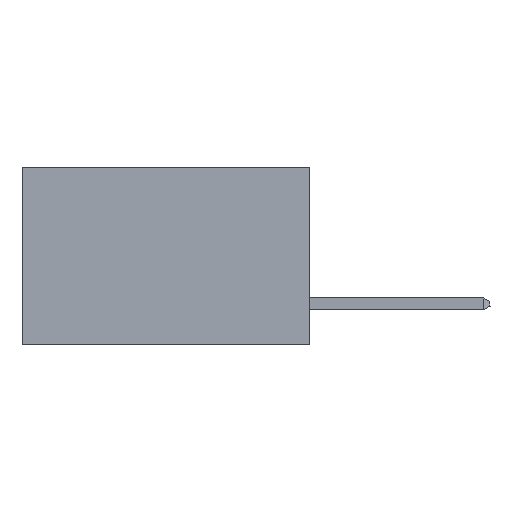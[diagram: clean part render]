
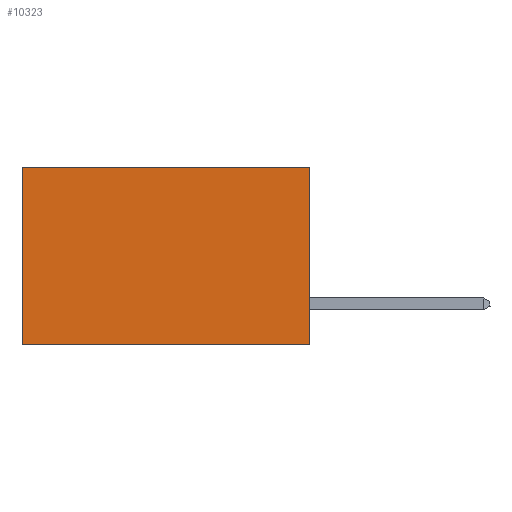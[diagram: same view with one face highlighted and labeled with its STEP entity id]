
A CAD part, left-side view. The second image highlights one B-rep face of the part: STEP entity #10323.
In plain terms, the highlighted planar face has unit normal (-1, 0, 0).
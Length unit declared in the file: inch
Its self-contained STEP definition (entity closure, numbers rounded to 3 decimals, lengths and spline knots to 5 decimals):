
#1846 = CARTESIAN_POINT ( 'NONE',  ( 0.2875, 0.6, 0. ) ) ;
#3329 = VECTOR ( 'NONE', #15902, 39.37008 ) ;
#3577 = CARTESIAN_POINT ( 'NONE',  ( 0.2875, 0.6, 0. ) ) ;
#4540 = EDGE_CURVE ( 'NONE', #26528, #11349, #8530, .T. ) ;
#5755 = FACE_OUTER_BOUND ( 'NONE', #14422, .T. ) ;
#8501 = VERTEX_POINT ( 'NONE', #25374 ) ;
#8530 = LINE ( 'NONE', #32271, #3329 ) ;
#8565 = ORIENTED_EDGE ( 'NONE', *, *, #35261, .F. ) ;
#10323 = ADVANCED_FACE ( 'NONE', ( #5755 ), #11440, .F. ) ;
#10824 = VECTOR ( 'NONE', #27989, 39.37008 ) ;
#11349 = VERTEX_POINT ( 'NONE', #3577 ) ;
#11440 = PLANE ( 'NONE',  #23924 ) ;
#12694 = ORIENTED_EDGE ( 'NONE', *, *, #17132, .T. ) ;
#13434 = ORIENTED_EDGE ( 'NONE', *, *, #30711, .F. ) ;
#13643 = LINE ( 'NONE', #32342, #16226 ) ;
#14422 = EDGE_LOOP ( 'NONE', ( #12694, #8565, #13434, #18139 ) ) ;
#14729 = CARTESIAN_POINT ( 'NONE',  ( 0.2875, 0., -0.37 ) ) ;
#15571 = LINE ( 'NONE', #14729, #10824 ) ;
#15708 = DIRECTION ( 'NONE',  ( 0., 0., -1. ) ) ;
#15902 = DIRECTION ( 'NONE',  ( 0., 1., 0. ) ) ;
#16226 = VECTOR ( 'NONE', #17723, 39.37008 ) ;
#17132 = EDGE_CURVE ( 'NONE', #11349, #22255, #30994, .T. ) ;
#17723 = DIRECTION ( 'NONE',  ( 0., 0., -1. ) ) ;
#18139 = ORIENTED_EDGE ( 'NONE', *, *, #4540, .T. ) ;
#19600 = CARTESIAN_POINT ( 'NONE',  ( 0.2875, 0., 0. ) ) ;
#20418 = CARTESIAN_POINT ( 'NONE',  ( 0.2875, 0.6, -0.37 ) ) ;
#22255 = VERTEX_POINT ( 'NONE', #20418 ) ;
#23924 = AXIS2_PLACEMENT_3D ( 'NONE', #33978, #33484, #33738 ) ;
#25374 = CARTESIAN_POINT ( 'NONE',  ( 0.2875, 0., -0.37 ) ) ;
#26528 = VERTEX_POINT ( 'NONE', #19600 ) ;
#27989 = DIRECTION ( 'NONE',  ( 0., 1., 0. ) ) ;
#28407 = VECTOR ( 'NONE', #15708, 39.37008 ) ;
#30711 = EDGE_CURVE ( 'NONE', #26528, #8501, #13643, .T. ) ;
#30994 = LINE ( 'NONE', #1846, #28407 ) ;
#32271 = CARTESIAN_POINT ( 'NONE',  ( 0.2875, 0., 0. ) ) ;
#32342 = CARTESIAN_POINT ( 'NONE',  ( 0.2875, 0., 0. ) ) ;
#33484 = DIRECTION ( 'NONE',  ( 1., 0., 0. ) ) ;
#33738 = DIRECTION ( 'NONE',  ( 0., 0., -1. ) ) ;
#33978 = CARTESIAN_POINT ( 'NONE',  ( 0.2875, 0., 0. ) ) ;
#35261 = EDGE_CURVE ( 'NONE', #8501, #22255, #15571, .T. ) ;
